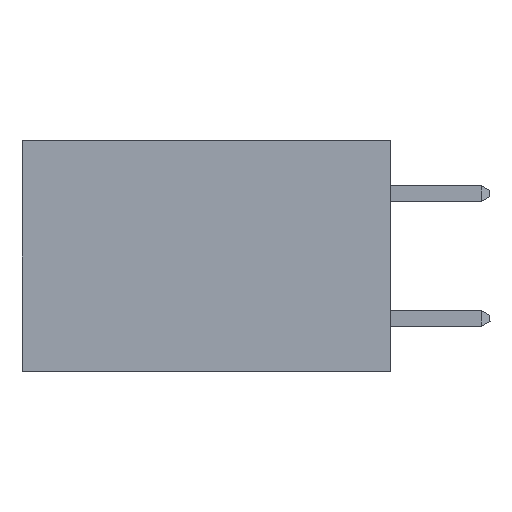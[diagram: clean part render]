
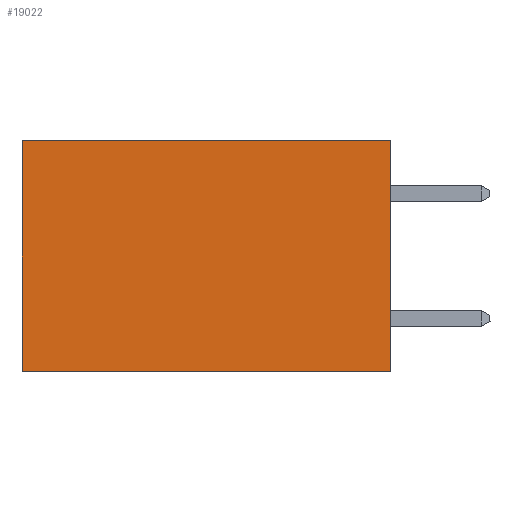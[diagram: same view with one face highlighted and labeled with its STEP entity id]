
A CAD part, left-side view. The second image highlights one B-rep face of the part: STEP entity #19022.
In plain terms, the highlighted planar face has unit normal (-1, 0, 0).
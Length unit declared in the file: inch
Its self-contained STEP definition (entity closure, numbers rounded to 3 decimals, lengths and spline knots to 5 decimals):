
#363 = EDGE_CURVE ( 'NONE', #27418, #24924, #605, .T. ) ;
#473 = CARTESIAN_POINT ( 'NONE',  ( 0.277, 0.59, -0.37 ) ) ;
#505 = PLANE ( 'NONE',  #10470 ) ;
#599 = DIRECTION ( 'NONE',  ( 0., 0., -1. ) ) ;
#605 = LINE ( 'NONE', #22101, #23551 ) ;
#2656 = LINE ( 'NONE', #473, #8644 ) ;
#2739 = DIRECTION ( 'NONE',  ( 1., 0., 0. ) ) ;
#4709 = VERTEX_POINT ( 'NONE', #19382 ) ;
#6027 = ORIENTED_EDGE ( 'NONE', *, *, #363, .T. ) ;
#7920 = EDGE_CURVE ( 'NONE', #24924, #4709, #2656, .T. ) ;
#8644 = VECTOR ( 'NONE', #599, 39.37008 ) ;
#9250 = FACE_OUTER_BOUND ( 'NONE', #27901, .T. ) ;
#9628 = CARTESIAN_POINT ( 'NONE',  ( 0.277, 0.59, 0. ) ) ;
#9679 = ORIENTED_EDGE ( 'NONE', *, *, #7920, .T. ) ;
#10470 = AXIS2_PLACEMENT_3D ( 'NONE', #18117, #2739, #18306 ) ;
#10577 = LINE ( 'NONE', #11784, #17179 ) ;
#11572 = ORIENTED_EDGE ( 'NONE', *, *, #26257, .F. ) ;
#11784 = CARTESIAN_POINT ( 'NONE',  ( 0.277, 0., -0.37 ) ) ;
#13236 = DIRECTION ( 'NONE',  ( 0., 0., -1. ) ) ;
#14561 = ORIENTED_EDGE ( 'NONE', *, *, #26708, .F. ) ;
#15437 = CARTESIAN_POINT ( 'NONE',  ( 0.277, 0., -0.37 ) ) ;
#15453 = CARTESIAN_POINT ( 'NONE',  ( 0.277, 0., 0. ) ) ;
#15750 = LINE ( 'NONE', #26480, #16444 ) ;
#16444 = VECTOR ( 'NONE', #13236, 39.37008 ) ;
#16861 = VERTEX_POINT ( 'NONE', #15437 ) ;
#17179 = VECTOR ( 'NONE', #25045, 39.37008 ) ;
#18117 = CARTESIAN_POINT ( 'NONE',  ( 0.277, 0., -0.37 ) ) ;
#18306 = DIRECTION ( 'NONE',  ( 0., 0., -1. ) ) ;
#19022 = ADVANCED_FACE ( 'NONE', ( #9250 ), #505, .F. ) ;
#19382 = CARTESIAN_POINT ( 'NONE',  ( 0.277, 0.59, -0.37 ) ) ;
#20936 = DIRECTION ( 'NONE',  ( 0., 1., 0. ) ) ;
#22101 = CARTESIAN_POINT ( 'NONE',  ( 0.277, 0., 0. ) ) ;
#23551 = VECTOR ( 'NONE', #20936, 39.37008 ) ;
#24924 = VERTEX_POINT ( 'NONE', #9628 ) ;
#25045 = DIRECTION ( 'NONE',  ( 0., 1., 0. ) ) ;
#26257 = EDGE_CURVE ( 'NONE', #16861, #4709, #10577, .T. ) ;
#26480 = CARTESIAN_POINT ( 'NONE',  ( 0.277, 0., -0.37 ) ) ;
#26708 = EDGE_CURVE ( 'NONE', #27418, #16861, #15750, .T. ) ;
#27418 = VERTEX_POINT ( 'NONE', #15453 ) ;
#27901 = EDGE_LOOP ( 'NONE', ( #9679, #11572, #14561, #6027 ) ) ;
